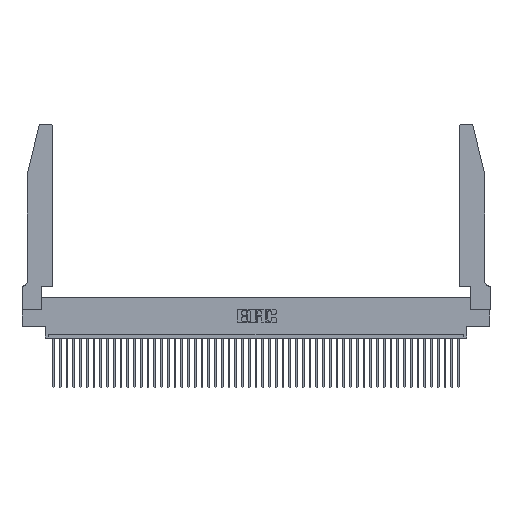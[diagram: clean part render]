
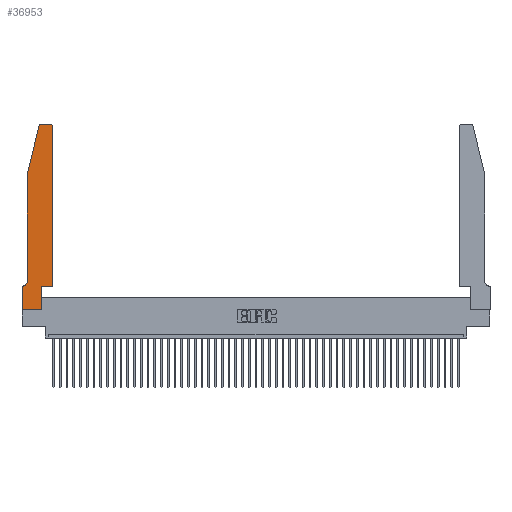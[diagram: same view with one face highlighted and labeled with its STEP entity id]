
A CAD part, top view. The second image highlights one B-rep face of the part: STEP entity #36953.
In plain terms, the highlighted planar face has unit normal (0, 0, 1).
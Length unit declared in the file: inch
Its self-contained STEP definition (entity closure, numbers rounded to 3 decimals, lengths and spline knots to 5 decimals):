
#783 = CARTESIAN_POINT ( 'NONE',  ( 0.0055, 0.42, 0.37 ) ) ;
#1934 = CARTESIAN_POINT ( 'NONE',  ( 0.284, 2.75, 0.37 ) ) ;
#2379 = CARTESIAN_POINT ( 'NONE',  ( 0.2865, 0.35, 0.37 ) ) ;
#3788 = VECTOR ( 'NONE', #21991, 39.37008 ) ;
#4002 = ORIENTED_EDGE ( 'NONE', *, *, #8143, .T. ) ;
#4348 = DIRECTION ( 'NONE',  ( 1., 0., 0. ) ) ;
#4409 = DIRECTION ( 'NONE',  ( 0., 0., -1. ) ) ;
#4444 = CARTESIAN_POINT ( 'NONE',  ( 0.4205, 2.75, 0.37 ) ) ;
#5043 = AXIS2_PLACEMENT_3D ( 'NONE', #783, #4409, #30159 ) ;
#5186 = ORIENTED_EDGE ( 'NONE', *, *, #20939, .T. ) ;
#5306 = VERTEX_POINT ( 'NONE', #41732 ) ;
#5345 = DIRECTION ( 'NONE',  ( -0.239, -0.971, 0. ) ) ;
#6342 = VERTEX_POINT ( 'NONE', #7768 ) ;
#6987 = CIRCLE ( 'NONE', #5043, 0.07 ) ;
#7158 = EDGE_LOOP ( 'NONE', ( #38138, #16375, #24077, #5186, #18124, #20707, #7596, #12262, #38694, #36113, #4002, #24335 ) ) ;
#7596 = ORIENTED_EDGE ( 'NONE', *, *, #15331, .T. ) ;
#7604 = CARTESIAN_POINT ( 'NONE',  ( 0.4205, 2.72, 0.37 ) ) ;
#7768 = CARTESIAN_POINT ( 'NONE',  ( 0.4505, 2.72, 0.37 ) ) ;
#8143 = EDGE_CURVE ( 'NONE', #38030, #6342, #39482, .T. ) ;
#8451 = LINE ( 'NONE', #44334, #3788 ) ;
#8604 = AXIS2_PLACEMENT_3D ( 'NONE', #45546, #34274, #38233 ) ;
#8721 = VECTOR ( 'NONE', #22339, 39.37008 ) ;
#8871 = DIRECTION ( 'NONE',  ( -1., 0., 0. ) ) ;
#8909 = DIRECTION ( 'NONE',  ( 1., 0., 0. ) ) ;
#10002 = CARTESIAN_POINT ( 'NONE',  ( 0.0755, 0.42, 0.37 ) ) ;
#10569 = LINE ( 'NONE', #12271, #15195 ) ;
#12262 = ORIENTED_EDGE ( 'NONE', *, *, #15417, .T. ) ;
#12271 = CARTESIAN_POINT ( 'NONE',  ( 0.2605, 2.75, 0.37 ) ) ;
#12754 = CARTESIAN_POINT ( 'NONE',  ( 0.4505, 0.35, 0.37 ) ) ;
#13350 = LINE ( 'NONE', #14865, #8721 ) ;
#13382 = VECTOR ( 'NONE', #15801, 39.37008 ) ;
#13821 = EDGE_CURVE ( 'NONE', #28305, #36377, #10569, .T. ) ;
#14865 = CARTESIAN_POINT ( 'NONE',  ( 0.0755, 2., 0.37 ) ) ;
#15195 = VECTOR ( 'NONE', #8871, 39.37008 ) ;
#15331 = EDGE_CURVE ( 'NONE', #42478, #40361, #18098, .T. ) ;
#15417 = EDGE_CURVE ( 'NONE', #40361, #22711, #25601, .T. ) ;
#15801 = DIRECTION ( 'NONE',  ( 1., 0., 0. ) ) ;
#16020 = FACE_OUTER_BOUND ( 'NONE', #7158, .T. ) ;
#16375 = ORIENTED_EDGE ( 'NONE', *, *, #34226, .T. ) ;
#17102 = EDGE_CURVE ( 'NONE', #5306, #38030, #8451, .T. ) ;
#17581 = VERTEX_POINT ( 'NONE', #19471 ) ;
#17771 = VERTEX_POINT ( 'NONE', #25198 ) ;
#18098 = LINE ( 'NONE', #36800, #25646 ) ;
#18124 = ORIENTED_EDGE ( 'NONE', *, *, #41789, .T. ) ;
#18355 = CARTESIAN_POINT ( 'NONE',  ( 0.0755, 0.35, 0.37 ) ) ;
#19471 = CARTESIAN_POINT ( 'NONE',  ( 0.25487, 2.72718, 0.37 ) ) ;
#19613 = VECTOR ( 'NONE', #32213, 39.37008 ) ;
#19633 = VECTOR ( 'NONE', #41886, 39.37008 ) ;
#20707 = ORIENTED_EDGE ( 'NONE', *, *, #26689, .T. ) ;
#20939 = EDGE_CURVE ( 'NONE', #17771, #47939, #13350, .T. ) ;
#21991 = DIRECTION ( 'NONE',  ( 1., 0., 0. ) ) ;
#22280 = CARTESIAN_POINT ( 'NONE',  ( 0.2865, 0., 0.37 ) ) ;
#22339 = DIRECTION ( 'NONE',  ( 0., -1., 0. ) ) ;
#22343 = VECTOR ( 'NONE', #31347, 39.37008 ) ;
#22596 = VERTEX_POINT ( 'NONE', #46056 ) ;
#22711 = VERTEX_POINT ( 'NONE', #22280 ) ;
#24077 = ORIENTED_EDGE ( 'NONE', *, *, #27430, .T. ) ;
#24335 = ORIENTED_EDGE ( 'NONE', *, *, #45762, .T. ) ;
#24387 = CIRCLE ( 'NONE', #8604, 0.03 ) ;
#25198 = CARTESIAN_POINT ( 'NONE',  ( 0.0755, 2., 0.37 ) ) ;
#25601 = LINE ( 'NONE', #38157, #13382 ) ;
#25646 = VECTOR ( 'NONE', #41703, 39.37008 ) ;
#25648 = EDGE_CURVE ( 'NONE', #22711, #5306, #35946, .T. ) ;
#26689 = EDGE_CURVE ( 'NONE', #22596, #42478, #32299, .T. ) ;
#27430 = EDGE_CURVE ( 'NONE', #17581, #17771, #39238, .T. ) ;
#28305 = VERTEX_POINT ( 'NONE', #4444 ) ;
#29299 = VECTOR ( 'NONE', #5345, 39.37008 ) ;
#30159 = DIRECTION ( 'NONE',  ( -1., 0., 0. ) ) ;
#31250 = CARTESIAN_POINT ( 'NONE',  ( 0.0755, 2., 0.37 ) ) ;
#31347 = DIRECTION ( 'NONE',  ( -1., 0., 0. ) ) ;
#31562 = CARTESIAN_POINT ( 'NONE',  ( 0., 0.35, 0.37 ) ) ;
#32213 = DIRECTION ( 'NONE',  ( 0., 1., 0. ) ) ;
#32299 = LINE ( 'NONE', #18355, #22343 ) ;
#34226 = EDGE_CURVE ( 'NONE', #36377, #17581, #24387, .T. ) ;
#34274 = DIRECTION ( 'NONE',  ( 0., 0., 1. ) ) ;
#35443 = CARTESIAN_POINT ( 'NONE',  ( 0., 0., 0.37 ) ) ;
#35946 = LINE ( 'NONE', #2379, #19613 ) ;
#36113 = ORIENTED_EDGE ( 'NONE', *, *, #17102, .T. ) ;
#36377 = VERTEX_POINT ( 'NONE', #1934 ) ;
#36800 = CARTESIAN_POINT ( 'NONE',  ( 0., 0., 0.37 ) ) ;
#36953 = ADVANCED_FACE ( 'NONE', ( #16020 ), #42605, .T. ) ;
#37453 = DIRECTION ( 'NONE',  ( 0., 0., 1. ) ) ;
#38030 = VERTEX_POINT ( 'NONE', #12754 ) ;
#38138 = ORIENTED_EDGE ( 'NONE', *, *, #13821, .T. ) ;
#38157 = CARTESIAN_POINT ( 'NONE',  ( 0., 0., 0.37 ) ) ;
#38233 = DIRECTION ( 'NONE',  ( 1., 0., 0. ) ) ;
#38676 = AXIS2_PLACEMENT_3D ( 'NONE', #31562, #46354, #8909 ) ;
#38694 = ORIENTED_EDGE ( 'NONE', *, *, #25648, .T. ) ;
#38880 = CIRCLE ( 'NONE', #45397, 0.03 ) ;
#39238 = LINE ( 'NONE', #31250, #29299 ) ;
#39482 = LINE ( 'NONE', #40647, #19633 ) ;
#40361 = VERTEX_POINT ( 'NONE', #35443 ) ;
#40647 = CARTESIAN_POINT ( 'NONE',  ( 0.4505, 0.35, 0.37 ) ) ;
#41703 = DIRECTION ( 'NONE',  ( 0., -1., 0. ) ) ;
#41732 = CARTESIAN_POINT ( 'NONE',  ( 0.2865, 0.35, 0.37 ) ) ;
#41789 = EDGE_CURVE ( 'NONE', #47939, #22596, #6987, .T. ) ;
#41886 = DIRECTION ( 'NONE',  ( 0., 1., 0. ) ) ;
#42478 = VERTEX_POINT ( 'NONE', #44940 ) ;
#42605 = PLANE ( 'NONE',  #38676 ) ;
#44334 = CARTESIAN_POINT ( 'NONE',  ( 0.4505, 0.35, 0.37 ) ) ;
#44940 = CARTESIAN_POINT ( 'NONE',  ( 0., 0.35, 0.37 ) ) ;
#45397 = AXIS2_PLACEMENT_3D ( 'NONE', #7604, #37453, #4348 ) ;
#45546 = CARTESIAN_POINT ( 'NONE',  ( 0.284, 2.72, 0.37 ) ) ;
#45762 = EDGE_CURVE ( 'NONE', #6342, #28305, #38880, .T. ) ;
#46056 = CARTESIAN_POINT ( 'NONE',  ( 0.0055, 0.35, 0.37 ) ) ;
#46354 = DIRECTION ( 'NONE',  ( 0., 0., 1. ) ) ;
#47939 = VERTEX_POINT ( 'NONE', #10002 ) ;
